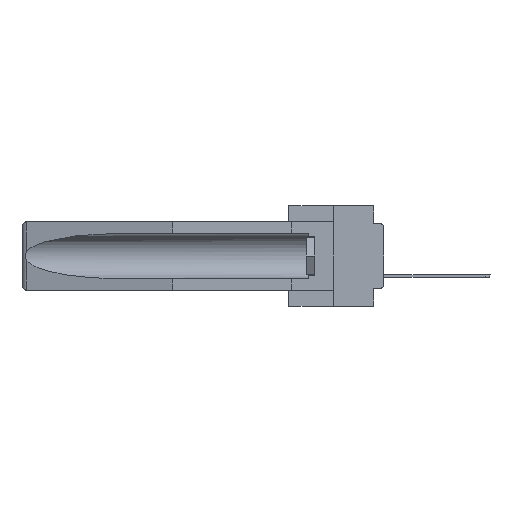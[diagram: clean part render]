
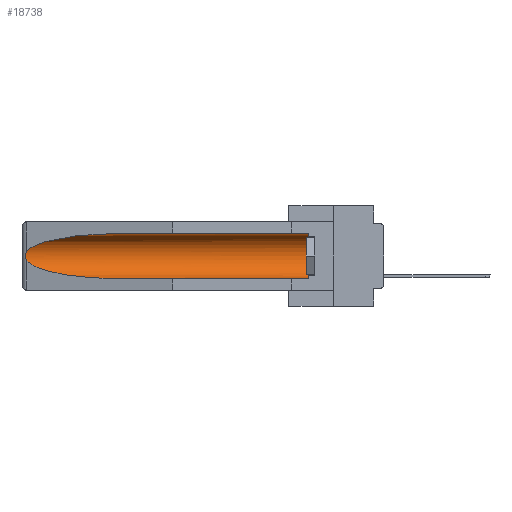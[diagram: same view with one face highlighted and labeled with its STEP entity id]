
A CAD part, left-side view. The second image highlights one B-rep face of the part: STEP entity #18738.
In plain terms, the highlighted cylindrical face has radius 2.857 mm (diameter 5.715 mm), a partial arc.
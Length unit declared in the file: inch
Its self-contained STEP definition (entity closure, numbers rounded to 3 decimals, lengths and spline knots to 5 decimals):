
#240 = EDGE_LOOP ( 'NONE', ( #23889, #3255, #28044, #3799, #24211, #24453 ) ) ;
#2024 = CARTESIAN_POINT ( 'NONE',  ( 0.155, -0.30754, -0.284 ) ) ;
#2094 = EDGE_CURVE ( 'NONE', #10791, #4471, #5123, .T. ) ;
#2183 = CARTESIAN_POINT ( 'NONE',  ( 0.26654, 1.53092, -0.15636 ) ) ;
#2388 = VERTEX_POINT ( 'NONE', #15465 ) ;
#2640 = CARTESIAN_POINT ( 'NONE',  ( 0.155, 0.126, -0.059 ) ) ;
#3255 = ORIENTED_EDGE ( 'NONE', *, *, #5391, .T. ) ;
#3498 = VECTOR ( 'NONE', #12772, 39.37008 ) ;
#3748 = VERTEX_POINT ( 'NONE', #2640 ) ;
#3799 = ORIENTED_EDGE ( 'NONE', *, *, #7128, .F. ) ;
#4471 = VERTEX_POINT ( 'NONE', #25290 ) ;
#5123 =( BOUNDED_CURVE ( )  B_SPLINE_CURVE ( 3, ( #23197, #9842, #25421, #27653 ),
 .UNSPECIFIED., .F., .F. ) 
 B_SPLINE_CURVE_WITH_KNOTS ( ( 4, 4 ),
 ( 0.1948, 1.5708 ),
 .UNSPECIFIED. ) 
 CURVE ( )  GEOMETRIC_REPRESENTATION_ITEM ( )  RATIONAL_B_SPLINE_CURVE ( ( 1., 0.848, 0.848, 1. ) ) 
 REPRESENTATION_ITEM ( '' )  );
#5391 = EDGE_CURVE ( 'NONE', #20635, #10791, #26202, .T. ) ;
#5789 = DIRECTION ( 'NONE',  ( 0., -1., 0. ) ) ;
#6545 = CARTESIAN_POINT ( 'NONE',  ( 0.2673, 1.53269, -0.17917 ) ) ;
#6576 = AXIS2_PLACEMENT_3D ( 'NONE', #10591, #5789, #14674 ) ;
#7128 = EDGE_CURVE ( 'NONE', #23581, #4471, #9194, .T. ) ;
#8080 = CARTESIAN_POINT ( 'NONE',  ( 0.26537, 1.52718, -0.14972 ) ) ;
#8231 = EDGE_CURVE ( 'NONE', #3748, #2388, #9780, .T. ) ;
#8449 = DIRECTION ( 'NONE',  ( 0., 1., 0. ) ) ;
#8503 = VECTOR ( 'NONE', #8449, 39.37008 ) ;
#9194 = LINE ( 'NONE', #2024, #8503 ) ;
#9780 = LINE ( 'NONE', #26100, #3498 ) ;
#9842 = CARTESIAN_POINT ( 'NONE',  ( 0.25451, 1.48313, -0.24835 ) ) ;
#10591 = CARTESIAN_POINT ( 'NONE',  ( 0.155, 0.126, -0.1715 ) ) ;
#10791 = VERTEX_POINT ( 'NONE', #17647 ) ;
#12120 = CARTESIAN_POINT ( 'NONE',  ( 0.26537, 1.52718, -0.14972 ) ) ;
#12772 = DIRECTION ( 'NONE',  ( 0., 1., 0. ) ) ;
#13209 = CARTESIAN_POINT ( 'NONE',  ( 0.26597, 1.52961, -0.15275 ) ) ;
#13311 = CARTESIAN_POINT ( 'NONE',  ( 0.26655, 1.53094, -0.18657 ) ) ;
#13866 = EDGE_CURVE ( 'NONE', #2388, #20635, #21565, .T. ) ;
#14674 = DIRECTION ( 'NONE',  ( 0., 0., 1. ) ) ;
#15381 = FACE_OUTER_BOUND ( 'NONE', #240, .T. ) ;
#15465 = CARTESIAN_POINT ( 'NONE',  ( 0.155, 1.07973, -0.059 ) ) ;
#17480 = DIRECTION ( 'NONE',  ( 0., 0., 1. ) ) ;
#17647 = CARTESIAN_POINT ( 'NONE',  ( 0.26537, 1.52718, -0.19328 ) ) ;
#17777 = CARTESIAN_POINT ( 'NONE',  ( 0.26597, 1.5296, -0.19026 ) ) ;
#18738 = ADVANCED_FACE ( 'NONE', ( #15381 ), #25855, .F. ) ;
#19207 = CARTESIAN_POINT ( 'NONE',  ( 0.25451, 1.48313, -0.09465 ) ) ;
#19448 = CIRCLE ( 'NONE', #6576, 0.1125 ) ;
#19937 = CARTESIAN_POINT ( 'NONE',  ( 0.2675, 1.53308, -0.17534 ) ) ;
#20022 = CARTESIAN_POINT ( 'NONE',  ( 0.155, -0.30754, -0.1715 ) ) ;
#20635 = VERTEX_POINT ( 'NONE', #12120 ) ;
#21549 = CARTESIAN_POINT ( 'NONE',  ( 0.21114, 1.30732, -0.059 ) ) ;
#21565 =( BOUNDED_CURVE ( )  B_SPLINE_CURVE ( 3, ( #25837, #21549, #19207, #8080 ),
 .UNSPECIFIED., .F., .F. ) 
 B_SPLINE_CURVE_WITH_KNOTS ( ( 4, 4 ),
 ( 4.71239, 6.08839 ),
 .UNSPECIFIED. ) 
 CURVE ( )  GEOMETRIC_REPRESENTATION_ITEM ( )  RATIONAL_B_SPLINE_CURVE ( ( 1., 0.848, 0.848, 1. ) ) 
 REPRESENTATION_ITEM ( '' )  );
#21875 = CARTESIAN_POINT ( 'NONE',  ( 0.2675, 1.53308, -0.16763 ) ) ;
#23111 = EDGE_CURVE ( 'NONE', #23581, #3748, #19448, .T. ) ;
#23197 = CARTESIAN_POINT ( 'NONE',  ( 0.26537, 1.52718, -0.19328 ) ) ;
#23581 = VERTEX_POINT ( 'NONE', #24256 ) ;
#23889 = ORIENTED_EDGE ( 'NONE', *, *, #13866, .T. ) ;
#24107 = CARTESIAN_POINT ( 'NONE',  ( 0.26537, 1.52718, -0.14972 ) ) ;
#24211 = ORIENTED_EDGE ( 'NONE', *, *, #23111, .T. ) ;
#24256 = CARTESIAN_POINT ( 'NONE',  ( 0.155, 0.126, -0.284 ) ) ;
#24453 = ORIENTED_EDGE ( 'NONE', *, *, #8231, .T. ) ;
#24484 = DIRECTION ( 'NONE',  ( 0., 1., 0. ) ) ;
#24788 = AXIS2_PLACEMENT_3D ( 'NONE', #20022, #24484, #17480 ) ;
#25290 = CARTESIAN_POINT ( 'NONE',  ( 0.155, 1.07973, -0.284 ) ) ;
#25421 = CARTESIAN_POINT ( 'NONE',  ( 0.21114, 1.30732, -0.284 ) ) ;
#25837 = CARTESIAN_POINT ( 'NONE',  ( 0.155, 1.07973, -0.059 ) ) ;
#25855 = CYLINDRICAL_SURFACE ( 'NONE', #24788, 0.1125 ) ;
#26100 = CARTESIAN_POINT ( 'NONE',  ( 0.155, -0.30754, -0.059 ) ) ;
#26202 = B_SPLINE_CURVE_WITH_KNOTS ( 'NONE', 3,
 ( #24107, #13209, #2183, #26624, #21875, #19937, #6545, #13311, #17777, #28870 ),
 .UNSPECIFIED., .F., .F.,
 ( 4, 2, 2, 2, 4 ),
 ( 0., 0.00029, 0.00058, 0.00087, 0.00117 ),
 .UNSPECIFIED. ) ;
#26624 = CARTESIAN_POINT ( 'NONE',  ( 0.2673, 1.5327, -0.16383 ) ) ;
#27653 = CARTESIAN_POINT ( 'NONE',  ( 0.155, 1.07973, -0.284 ) ) ;
#28044 = ORIENTED_EDGE ( 'NONE', *, *, #2094, .T. ) ;
#28870 = CARTESIAN_POINT ( 'NONE',  ( 0.26537, 1.52718, -0.19328 ) ) ;
